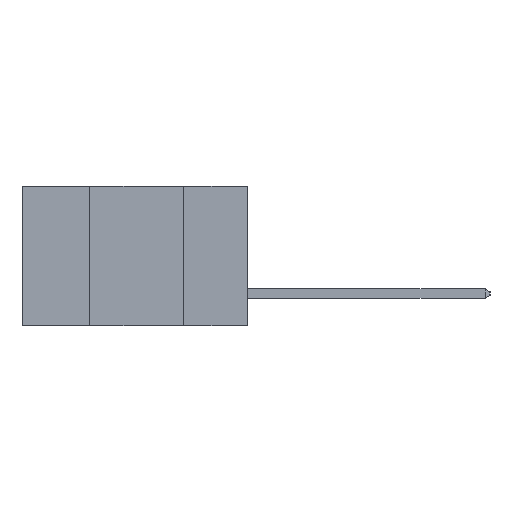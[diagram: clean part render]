
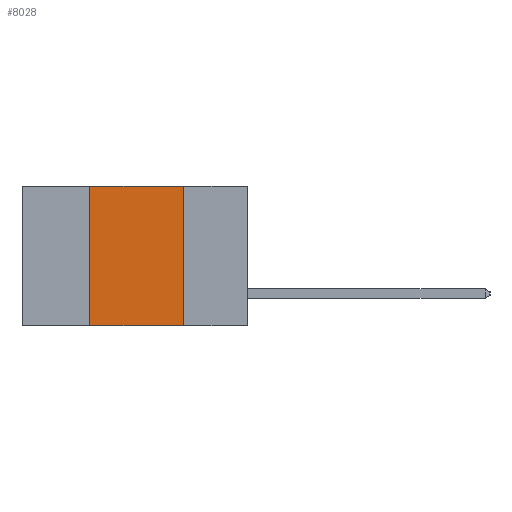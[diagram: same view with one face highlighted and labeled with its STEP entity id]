
A CAD part, left-side view. The second image highlights one B-rep face of the part: STEP entity #8028.
In plain terms, the highlighted planar face has unit normal (-1, 0, 0).
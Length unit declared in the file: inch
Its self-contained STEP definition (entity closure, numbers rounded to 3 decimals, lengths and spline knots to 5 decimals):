
#21 = DIRECTION ( 'NONE',  ( 0., -1., 0. ) ) ;
#426 = LINE ( 'NONE', #3463, #15178 ) ;
#997 = CARTESIAN_POINT ( 'NONE',  ( 0., 0.17, -0.37 ) ) ;
#1449 = LINE ( 'NONE', #997, #15283 ) ;
#1585 = VERTEX_POINT ( 'NONE', #6080 ) ;
#1739 = DIRECTION ( 'NONE',  ( 0., -1., 0. ) ) ;
#2268 = FACE_OUTER_BOUND ( 'NONE', #12162, .T. ) ;
#2472 = EDGE_CURVE ( 'NONE', #1585, #9467, #1449, .T. ) ;
#3463 = CARTESIAN_POINT ( 'NONE',  ( 0., 0.6, 0. ) ) ;
#3551 = AXIS2_PLACEMENT_3D ( 'NONE', #4375, #12761, #10158 ) ;
#3875 = VECTOR ( 'NONE', #1739, 39.37008 ) ;
#4030 = VECTOR ( 'NONE', #5131, 39.37008 ) ;
#4176 = CARTESIAN_POINT ( 'NONE',  ( 0., 0.6, -0.37 ) ) ;
#4225 = ORIENTED_EDGE ( 'NONE', *, *, #8897, .F. ) ;
#4375 = CARTESIAN_POINT ( 'NONE',  ( 0., 0.6, 0. ) ) ;
#4855 = CARTESIAN_POINT ( 'NONE',  ( 0., 0.17, -0.37 ) ) ;
#5131 = DIRECTION ( 'NONE',  ( 0., 0., 1. ) ) ;
#5356 = LINE ( 'NONE', #6304, #4030 ) ;
#6080 = CARTESIAN_POINT ( 'NONE',  ( 0., 0.17, 0. ) ) ;
#6304 = CARTESIAN_POINT ( 'NONE',  ( 0., 0.42, -0.37 ) ) ;
#8028 = ADVANCED_FACE ( 'NONE', ( #2268 ), #15169, .F. ) ;
#8841 = VERTEX_POINT ( 'NONE', #14221 ) ;
#8897 = EDGE_CURVE ( 'NONE', #9000, #1585, #426, .T. ) ;
#9000 = VERTEX_POINT ( 'NONE', #12542 ) ;
#9467 = VERTEX_POINT ( 'NONE', #4855 ) ;
#10099 = ORIENTED_EDGE ( 'NONE', *, *, #10666, .T. ) ;
#10150 = ORIENTED_EDGE ( 'NONE', *, *, #12251, .F. ) ;
#10158 = DIRECTION ( 'NONE',  ( 0., 0., -1. ) ) ;
#10666 = EDGE_CURVE ( 'NONE', #8841, #9467, #13270, .T. ) ;
#12162 = EDGE_LOOP ( 'NONE', ( #12329, #4225, #10150, #10099 ) ) ;
#12251 = EDGE_CURVE ( 'NONE', #8841, #9000, #5356, .T. ) ;
#12329 = ORIENTED_EDGE ( 'NONE', *, *, #2472, .F. ) ;
#12542 = CARTESIAN_POINT ( 'NONE',  ( 0., 0.42, 0. ) ) ;
#12761 = DIRECTION ( 'NONE',  ( 1., 0., 0. ) ) ;
#13270 = LINE ( 'NONE', #4176, #3875 ) ;
#14221 = CARTESIAN_POINT ( 'NONE',  ( 0., 0.42, -0.37 ) ) ;
#15169 = PLANE ( 'NONE',  #3551 ) ;
#15178 = VECTOR ( 'NONE', #21, 39.37008 ) ;
#15283 = VECTOR ( 'NONE', #15372, 39.37008 ) ;
#15372 = DIRECTION ( 'NONE',  ( 0., 0., -1. ) ) ;
